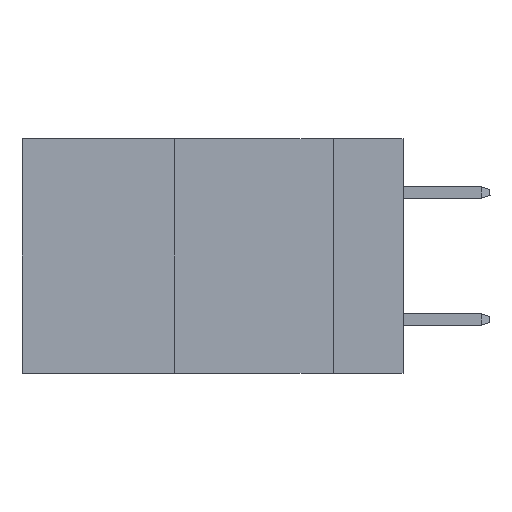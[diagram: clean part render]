
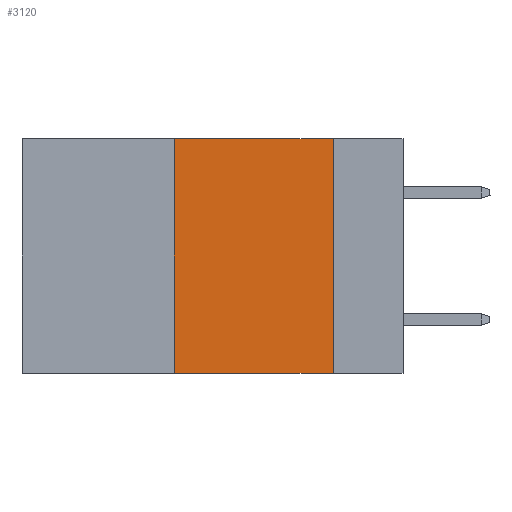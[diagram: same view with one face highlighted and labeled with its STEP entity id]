
A CAD part, left-side view. The second image highlights one B-rep face of the part: STEP entity #3120.
In plain terms, the highlighted planar face has unit normal (-1, 0, 0).
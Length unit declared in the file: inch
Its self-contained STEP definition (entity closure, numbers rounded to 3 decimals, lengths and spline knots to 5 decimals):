
#20 = VERTEX_POINT ( 'NONE', #7004 ) ;
#231 = ORIENTED_EDGE ( 'NONE', *, *, #3822, .F. ) ;
#330 = VECTOR ( 'NONE', #8002, 39.37008 ) ;
#446 = DIRECTION ( 'NONE',  ( 1., 0., 0. ) ) ;
#502 = VECTOR ( 'NONE', #1995, 39.37008 ) ;
#514 = VERTEX_POINT ( 'NONE', #560 ) ;
#560 = CARTESIAN_POINT ( 'NONE',  ( 0., 0.11, -0.37 ) ) ;
#1053 = DIRECTION ( 'NONE',  ( 0., 0., -1. ) ) ;
#1195 = CARTESIAN_POINT ( 'NONE',  ( 0., 0.6, 0. ) ) ;
#1351 = EDGE_CURVE ( 'NONE', #8429, #20, #3935, .T. ) ;
#1514 = LINE ( 'NONE', #3104, #5103 ) ;
#1995 = DIRECTION ( 'NONE',  ( 0., -1., 0. ) ) ;
#2023 = ORIENTED_EDGE ( 'NONE', *, *, #6976, .T. ) ;
#2613 = ORIENTED_EDGE ( 'NONE', *, *, #4339, .F. ) ;
#2685 = LINE ( 'NONE', #4988, #502 ) ;
#2742 = PLANE ( 'NONE',  #2848 ) ;
#2826 = LINE ( 'NONE', #4385, #330 ) ;
#2848 = AXIS2_PLACEMENT_3D ( 'NONE', #1195, #446, #1053 ) ;
#3104 = CARTESIAN_POINT ( 'NONE',  ( 0., 0.36, 0. ) ) ;
#3120 = ADVANCED_FACE ( 'NONE', ( #3294 ), #2742, .F. ) ;
#3247 = DIRECTION ( 'NONE',  ( 0., -1., 0. ) ) ;
#3294 = FACE_OUTER_BOUND ( 'NONE', #8136, .T. ) ;
#3822 = EDGE_CURVE ( 'NONE', #20, #514, #2826, .T. ) ;
#3935 = LINE ( 'NONE', #8376, #5930 ) ;
#4339 = EDGE_CURVE ( 'NONE', #6682, #8429, #1514, .T. ) ;
#4385 = CARTESIAN_POINT ( 'NONE',  ( 0., 0.11, 0. ) ) ;
#4988 = CARTESIAN_POINT ( 'NONE',  ( 0., 0.6, -0.37 ) ) ;
#5063 = ORIENTED_EDGE ( 'NONE', *, *, #1351, .F. ) ;
#5103 = VECTOR ( 'NONE', #6690, 39.37008 ) ;
#5930 = VECTOR ( 'NONE', #3247, 39.37008 ) ;
#6264 = CARTESIAN_POINT ( 'NONE',  ( 0., 0.36, 0. ) ) ;
#6616 = CARTESIAN_POINT ( 'NONE',  ( 0., 0.36, -0.37 ) ) ;
#6682 = VERTEX_POINT ( 'NONE', #6616 ) ;
#6690 = DIRECTION ( 'NONE',  ( 0., 0., 1. ) ) ;
#6976 = EDGE_CURVE ( 'NONE', #6682, #514, #2685, .T. ) ;
#7004 = CARTESIAN_POINT ( 'NONE',  ( 0., 0.11, 0. ) ) ;
#8002 = DIRECTION ( 'NONE',  ( 0., 0., -1. ) ) ;
#8136 = EDGE_LOOP ( 'NONE', ( #231, #5063, #2613, #2023 ) ) ;
#8376 = CARTESIAN_POINT ( 'NONE',  ( 0., 0.6, 0. ) ) ;
#8429 = VERTEX_POINT ( 'NONE', #6264 ) ;
